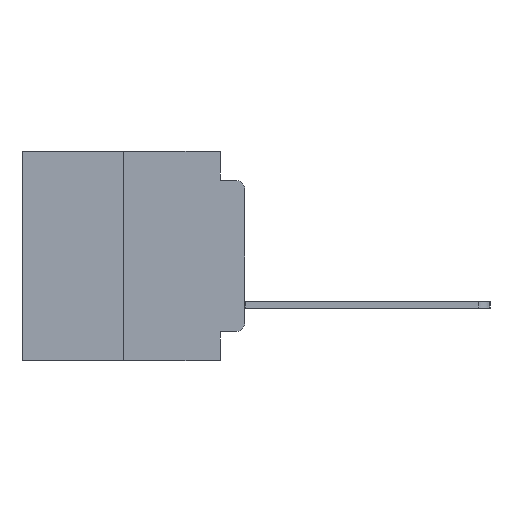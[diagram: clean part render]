
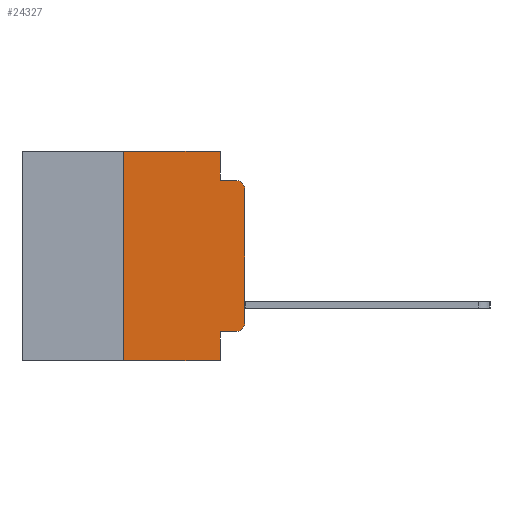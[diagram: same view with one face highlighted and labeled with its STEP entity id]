
A CAD part, left-side view. The second image highlights one B-rep face of the part: STEP entity #24327.
In plain terms, the highlighted planar face has unit normal (-1, 0, 0).
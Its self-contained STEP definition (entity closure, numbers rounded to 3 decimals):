
#119 = LINE ( 'NONE', #20461, #19378 ) ;
#177 = DIRECTION ( 'NONE',  ( 0., 0., 1. ) ) ;
#627 = CARTESIAN_POINT ( 'NONE',  ( -75.603, 1.295, -3.975 ) ) ;
#919 = ORIENTED_EDGE ( 'NONE', *, *, #26953, .T. ) ;
#1350 = ORIENTED_EDGE ( 'NONE', *, *, #11746, .T. ) ;
#1358 = ORIENTED_EDGE ( 'NONE', *, *, #9458, .F. ) ;
#1468 = CARTESIAN_POINT ( 'NONE',  ( -75.603, 0., -3.467 ) ) ;
#2182 = VERTEX_POINT ( 'NONE', #12161 ) ;
#2542 = CARTESIAN_POINT ( 'NONE',  ( -75.603, 0., 5.486 ) ) ;
#2590 = CARTESIAN_POINT ( 'NONE',  ( -75.603, 1.295, 0. ) ) ;
#2873 = LINE ( 'NONE', #18008, #5008 ) ;
#3099 = ORIENTED_EDGE ( 'NONE', *, *, #25148, .F. ) ;
#3109 = VERTEX_POINT ( 'NONE', #1468 ) ;
#3262 = VERTEX_POINT ( 'NONE', #13326 ) ;
#3267 = DIRECTION ( 'NONE',  ( -1., 0., 0. ) ) ;
#3291 = VECTOR ( 'NONE', #11369, 1000. ) ;
#3365 = DIRECTION ( 'NONE',  ( 0., 0., -1. ) ) ;
#3434 = EDGE_CURVE ( 'NONE', #10034, #24899, #21782, .T. ) ;
#3907 = EDGE_LOOP ( 'NONE', ( #919, #28425, #6637, #1350, #27781, #3099, #14551, #1358, #29384, #15084 ) ) ;
#3922 = DIRECTION ( 'NONE',  ( 0., 0., -1. ) ) ;
#4692 = EDGE_CURVE ( 'NONE', #3262, #10453, #119, .T. ) ;
#5008 = VECTOR ( 'NONE', #22227, 1000. ) ;
#5346 = VECTOR ( 'NONE', #177, 1000. ) ;
#5767 = CARTESIAN_POINT ( 'NONE',  ( -75.603, 1.295, -5.486 ) ) ;
#5870 = VERTEX_POINT ( 'NONE', #22948 ) ;
#5904 = DIRECTION ( 'NONE',  ( 1., 0., 0. ) ) ;
#6061 = AXIS2_PLACEMENT_3D ( 'NONE', #13067, #15395, #29300 ) ;
#6407 = VECTOR ( 'NONE', #14439, 1000. ) ;
#6436 = CIRCLE ( 'NONE', #7336, 0.508 ) ;
#6637 = ORIENTED_EDGE ( 'NONE', *, *, #13702, .T. ) ;
#7336 = AXIS2_PLACEMENT_3D ( 'NONE', #21735, #3267, #3365 ) ;
#8200 = CARTESIAN_POINT ( 'NONE',  ( -75.603, 11.684, 5.486 ) ) ;
#8549 = CARTESIAN_POINT ( 'NONE',  ( -75.603, 1.295, 5.486 ) ) ;
#8817 = CARTESIAN_POINT ( 'NONE',  ( -75.603, 1.295, 0. ) ) ;
#8860 = DIRECTION ( 'NONE',  ( 0., -1., 0. ) ) ;
#9012 = CIRCLE ( 'NONE', #6061, 0.508 ) ;
#9458 = EDGE_CURVE ( 'NONE', #10034, #3262, #17971, .T. ) ;
#10034 = VERTEX_POINT ( 'NONE', #29292 ) ;
#10453 = VERTEX_POINT ( 'NONE', #8549 ) ;
#11369 = DIRECTION ( 'NONE',  ( 0., 0., -1. ) ) ;
#11503 = AXIS2_PLACEMENT_3D ( 'NONE', #8200, #5904, #3922 ) ;
#11627 = DIRECTION ( 'NONE',  ( 0., -1., 0. ) ) ;
#11746 = EDGE_CURVE ( 'NONE', #2182, #17270, #9012, .T. ) ;
#11787 = VECTOR ( 'NONE', #11627, 1000. ) ;
#11902 = VECTOR ( 'NONE', #20621, 1000. ) ;
#11941 = CARTESIAN_POINT ( 'NONE',  ( -75.603, 1.295, 3.975 ) ) ;
#12161 = CARTESIAN_POINT ( 'NONE',  ( -75.603, 0., 3.467 ) ) ;
#13067 = CARTESIAN_POINT ( 'NONE',  ( -75.603, 0.508, 3.467 ) ) ;
#13188 = LINE ( 'NONE', #11941, #6407 ) ;
#13326 = CARTESIAN_POINT ( 'NONE',  ( -75.603, 6.35, 5.486 ) ) ;
#13702 = EDGE_CURVE ( 'NONE', #3109, #2182, #15015, .T. ) ;
#14048 = CARTESIAN_POINT ( 'NONE',  ( -75.603, 1.295, 3.975 ) ) ;
#14439 = DIRECTION ( 'NONE',  ( 0., -1., 0. ) ) ;
#14551 = ORIENTED_EDGE ( 'NONE', *, *, #4692, .F. ) ;
#14726 = LINE ( 'NONE', #2590, #3291 ) ;
#15015 = LINE ( 'NONE', #2542, #5346 ) ;
#15084 = ORIENTED_EDGE ( 'NONE', *, *, #20251, .F. ) ;
#15395 = DIRECTION ( 'NONE',  ( -1., 0., 0. ) ) ;
#15532 = DIRECTION ( 'NONE',  ( 0., 0., -1. ) ) ;
#17270 = VERTEX_POINT ( 'NONE', #22200 ) ;
#17516 = EDGE_CURVE ( 'NONE', #5870, #3109, #6436, .T. ) ;
#17601 = PLANE ( 'NONE',  #11503 ) ;
#17971 = LINE ( 'NONE', #27543, #11902 ) ;
#17993 = EDGE_CURVE ( 'NONE', #29477, #17270, #13188, .T. ) ;
#18008 = CARTESIAN_POINT ( 'NONE',  ( -75.603, 1.295, -3.975 ) ) ;
#19378 = VECTOR ( 'NONE', #8860, 1000. ) ;
#19562 = VECTOR ( 'NONE', #15532, 1000. ) ;
#20251 = EDGE_CURVE ( 'NONE', #23400, #24899, #20997, .T. ) ;
#20461 = CARTESIAN_POINT ( 'NONE',  ( -75.603, 11.684, 5.486 ) ) ;
#20621 = DIRECTION ( 'NONE',  ( 0., 0., 1. ) ) ;
#20997 = LINE ( 'NONE', #8817, #19562 ) ;
#21735 = CARTESIAN_POINT ( 'NONE',  ( -75.603, 0.508, -3.467 ) ) ;
#21782 = LINE ( 'NONE', #27559, #11787 ) ;
#22200 = CARTESIAN_POINT ( 'NONE',  ( -75.603, 0.508, 3.975 ) ) ;
#22227 = DIRECTION ( 'NONE',  ( 0., -1., 0. ) ) ;
#22948 = CARTESIAN_POINT ( 'NONE',  ( -75.603, 0.508, -3.975 ) ) ;
#23400 = VERTEX_POINT ( 'NONE', #627 ) ;
#24327 = ADVANCED_FACE ( 'NONE', ( #25451 ), #17601, .F. ) ;
#24899 = VERTEX_POINT ( 'NONE', #5767 ) ;
#25148 = EDGE_CURVE ( 'NONE', #10453, #29477, #14726, .T. ) ;
#25451 = FACE_OUTER_BOUND ( 'NONE', #3907, .T. ) ;
#26953 = EDGE_CURVE ( 'NONE', #23400, #5870, #2873, .T. ) ;
#27543 = CARTESIAN_POINT ( 'NONE',  ( -75.603, 6.35, -5.486 ) ) ;
#27559 = CARTESIAN_POINT ( 'NONE',  ( -75.603, 11.684, -5.486 ) ) ;
#27781 = ORIENTED_EDGE ( 'NONE', *, *, #17993, .F. ) ;
#28425 = ORIENTED_EDGE ( 'NONE', *, *, #17516, .T. ) ;
#29292 = CARTESIAN_POINT ( 'NONE',  ( -75.603, 6.35, -5.486 ) ) ;
#29300 = DIRECTION ( 'NONE',  ( 0., 0., -1. ) ) ;
#29384 = ORIENTED_EDGE ( 'NONE', *, *, #3434, .T. ) ;
#29477 = VERTEX_POINT ( 'NONE', #14048 ) ;
